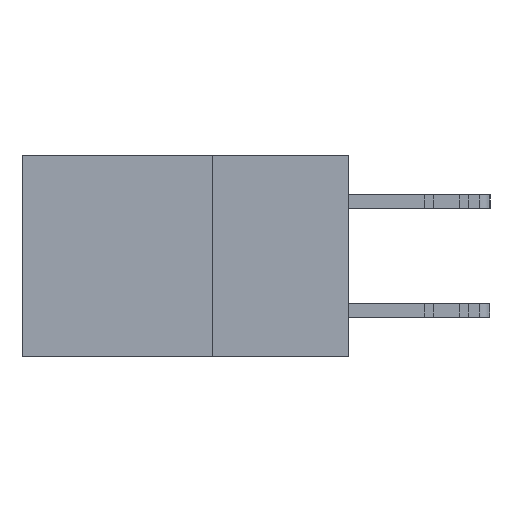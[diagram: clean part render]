
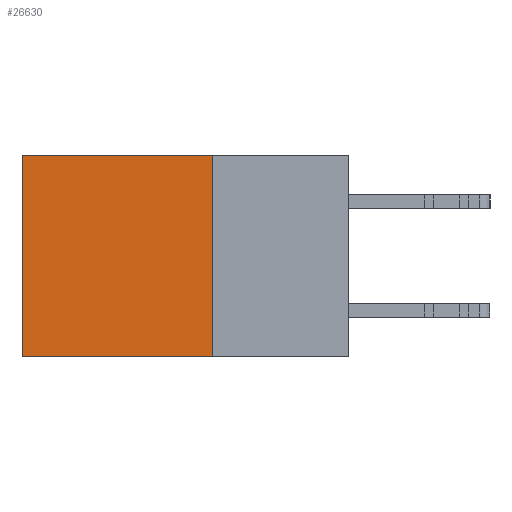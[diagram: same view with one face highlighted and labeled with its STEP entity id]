
A CAD part, left-side view. The second image highlights one B-rep face of the part: STEP entity #26630.
In plain terms, the highlighted planar face has unit normal (-1, 0, 0).
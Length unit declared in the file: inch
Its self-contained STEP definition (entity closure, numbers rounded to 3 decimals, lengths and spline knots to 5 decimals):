
#289 = VERTEX_POINT ( 'NONE', #12453 ) ;
#1160 = DIRECTION ( 'NONE',  ( 0., 0., -1. ) ) ;
#4677 = EDGE_CURVE ( 'NONE', #12826, #289, #15540, .T. ) ;
#4955 = CARTESIAN_POINT ( 'NONE',  ( 0.298, 0.25, 0. ) ) ;
#5485 = LINE ( 'NONE', #16357, #12236 ) ;
#5804 = AXIS2_PLACEMENT_3D ( 'NONE', #4955, #22625, #7538 ) ;
#6802 = VECTOR ( 'NONE', #11542, 39.37008 ) ;
#7538 = DIRECTION ( 'NONE',  ( 0., 0., -1. ) ) ;
#9214 = VECTOR ( 'NONE', #22304, 39.37008 ) ;
#9662 = VECTOR ( 'NONE', #10124, 39.37008 ) ;
#10124 = DIRECTION ( 'NONE',  ( 0., 0., -1. ) ) ;
#10381 = ORIENTED_EDGE ( 'NONE', *, *, #23480, .T. ) ;
#11542 = DIRECTION ( 'NONE',  ( 0., 1., 0. ) ) ;
#12236 = VECTOR ( 'NONE', #1160, 39.37008 ) ;
#12453 = CARTESIAN_POINT ( 'NONE',  ( 0.298, 0.25, -0.37 ) ) ;
#12826 = VERTEX_POINT ( 'NONE', #23208 ) ;
#14786 = EDGE_CURVE ( 'NONE', #289, #14891, #22612, .T. ) ;
#14891 = VERTEX_POINT ( 'NONE', #17667 ) ;
#15540 = LINE ( 'NONE', #30850, #9662 ) ;
#16231 = ORIENTED_EDGE ( 'NONE', *, *, #14786, .F. ) ;
#16357 = CARTESIAN_POINT ( 'NONE',  ( 0.298, 0.6, 0. ) ) ;
#17667 = CARTESIAN_POINT ( 'NONE',  ( 0.298, 0.6, -0.37 ) ) ;
#18464 = EDGE_LOOP ( 'NONE', ( #25828, #16231, #28047, #10381 ) ) ;
#18841 = EDGE_CURVE ( 'NONE', #21711, #14891, #5485, .T. ) ;
#21711 = VERTEX_POINT ( 'NONE', #30883 ) ;
#22304 = DIRECTION ( 'NONE',  ( 0., 1., 0. ) ) ;
#22612 = LINE ( 'NONE', #27267, #9214 ) ;
#22625 = DIRECTION ( 'NONE',  ( 1., 0., 0. ) ) ;
#23208 = CARTESIAN_POINT ( 'NONE',  ( 0.298, 0.25, 0. ) ) ;
#23480 = EDGE_CURVE ( 'NONE', #12826, #21711, #26083, .T. ) ;
#23928 = CARTESIAN_POINT ( 'NONE',  ( 0.298, 0.25, 0. ) ) ;
#25828 = ORIENTED_EDGE ( 'NONE', *, *, #18841, .T. ) ;
#26083 = LINE ( 'NONE', #23928, #6802 ) ;
#26630 = ADVANCED_FACE ( 'NONE', ( #30041 ), #29961, .F. ) ;
#27267 = CARTESIAN_POINT ( 'NONE',  ( 0.298, 0.25, -0.37 ) ) ;
#28047 = ORIENTED_EDGE ( 'NONE', *, *, #4677, .F. ) ;
#29961 = PLANE ( 'NONE',  #5804 ) ;
#30041 = FACE_OUTER_BOUND ( 'NONE', #18464, .T. ) ;
#30850 = CARTESIAN_POINT ( 'NONE',  ( 0.298, 0.25, 0. ) ) ;
#30883 = CARTESIAN_POINT ( 'NONE',  ( 0.298, 0.6, 0. ) ) ;
